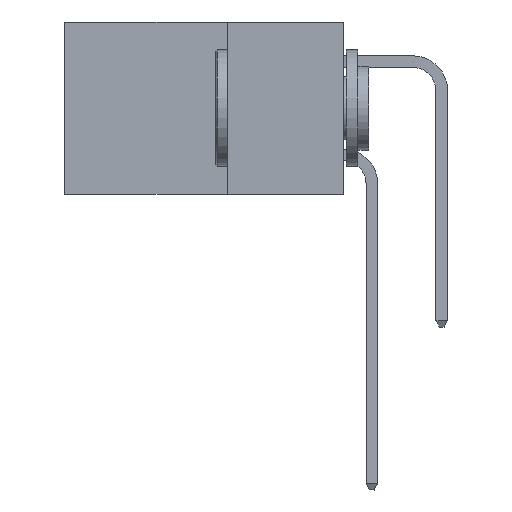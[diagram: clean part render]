
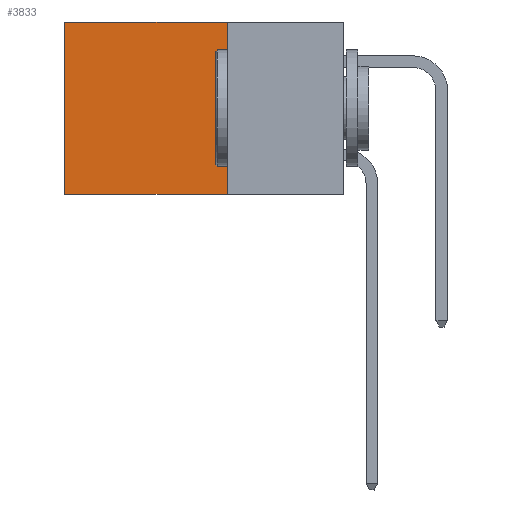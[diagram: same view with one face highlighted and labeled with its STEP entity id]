
A CAD part, left-side view. The second image highlights one B-rep face of the part: STEP entity #3833.
In plain terms, the highlighted planar face has unit normal (-1, 0, 0).
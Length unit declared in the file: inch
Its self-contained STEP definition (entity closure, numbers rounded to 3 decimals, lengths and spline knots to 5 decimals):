
#485 = LINE ( 'NONE', #12986, #14549 ) ;
#678 = LINE ( 'NONE', #10041, #11514 ) ;
#1369 = ORIENTED_EDGE ( 'NONE', *, *, #6532, .F. ) ;
#2229 = ORIENTED_EDGE ( 'NONE', *, *, #2654, .T. ) ;
#2654 = EDGE_CURVE ( 'NONE', #17329, #15843, #6604, .T. ) ;
#2812 = EDGE_CURVE ( 'NONE', #17329, #9607, #678, .T. ) ;
#3809 = CARTESIAN_POINT ( 'NONE',  ( 0.298, 0.25, 0. ) ) ;
#3833 = ADVANCED_FACE ( 'NONE', ( #14767 ), #15293, .F. ) ;
#5585 = CARTESIAN_POINT ( 'NONE',  ( 0.298, 0.6, -0.37 ) ) ;
#5940 = DIRECTION ( 'NONE',  ( 0., 0., -1. ) ) ;
#6532 = EDGE_CURVE ( 'NONE', #9607, #14486, #14023, .T. ) ;
#6604 = LINE ( 'NONE', #3809, #11285 ) ;
#7617 = CARTESIAN_POINT ( 'NONE',  ( 0.298, 0.25, -0.37 ) ) ;
#7823 = ORIENTED_EDGE ( 'NONE', *, *, #2812, .F. ) ;
#8444 = DIRECTION ( 'NONE',  ( 0., 0., -1. ) ) ;
#9607 = VERTEX_POINT ( 'NONE', #7617 ) ;
#10041 = CARTESIAN_POINT ( 'NONE',  ( 0.298, 0.25, 0. ) ) ;
#10272 = DIRECTION ( 'NONE',  ( 0., 1., 0. ) ) ;
#11285 = VECTOR ( 'NONE', #14993, 39.37008 ) ;
#11473 = AXIS2_PLACEMENT_3D ( 'NONE', #12672, #13910, #8444 ) ;
#11514 = VECTOR ( 'NONE', #12842, 39.37008 ) ;
#11938 = CARTESIAN_POINT ( 'NONE',  ( 0.298, 0.25, 0. ) ) ;
#12351 = ORIENTED_EDGE ( 'NONE', *, *, #13074, .T. ) ;
#12672 = CARTESIAN_POINT ( 'NONE',  ( 0.298, 0.25, 0. ) ) ;
#12842 = DIRECTION ( 'NONE',  ( 0., 0., -1. ) ) ;
#12986 = CARTESIAN_POINT ( 'NONE',  ( 0.298, 0.6, 0. ) ) ;
#13074 = EDGE_CURVE ( 'NONE', #15843, #14486, #485, .T. ) ;
#13910 = DIRECTION ( 'NONE',  ( 1., 0., 0. ) ) ;
#14023 = LINE ( 'NONE', #14776, #14685 ) ;
#14486 = VERTEX_POINT ( 'NONE', #5585 ) ;
#14549 = VECTOR ( 'NONE', #5940, 39.37008 ) ;
#14685 = VECTOR ( 'NONE', #10272, 39.37008 ) ;
#14767 = FACE_OUTER_BOUND ( 'NONE', #17927, .T. ) ;
#14776 = CARTESIAN_POINT ( 'NONE',  ( 0.298, 0.25, -0.37 ) ) ;
#14993 = DIRECTION ( 'NONE',  ( 0., 1., 0. ) ) ;
#15293 = PLANE ( 'NONE',  #11473 ) ;
#15843 = VERTEX_POINT ( 'NONE', #16311 ) ;
#16311 = CARTESIAN_POINT ( 'NONE',  ( 0.298, 0.6, 0. ) ) ;
#17329 = VERTEX_POINT ( 'NONE', #11938 ) ;
#17927 = EDGE_LOOP ( 'NONE', ( #12351, #1369, #7823, #2229 ) ) ;
